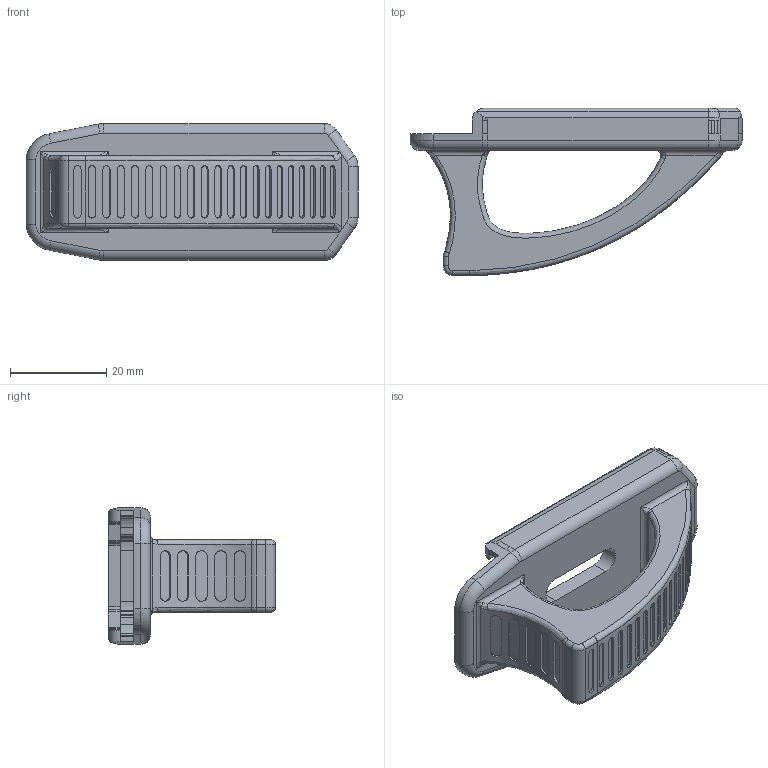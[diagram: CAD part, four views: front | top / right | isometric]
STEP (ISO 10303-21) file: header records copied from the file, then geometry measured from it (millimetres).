
FILE_DESCRIPTION (( 'STEP AP214' ), '1' );
FILE_NAME ('Ranger_Plate.STEP', '2022-09-24T15:52:26', ( '' ), ( '' ), 'SwSTEP 2.0', 'SolidWorks 2021', '' );
FILE_SCHEMA (( 'AUTOMOTIVE_DESIGN' ));
Length unit declared in the file: millimetre
Products named in the file (1): Ranger_Plate
Bounding box: 68.9 x 34.68 x 28.4 mm (x, y, z)
Volume: 15761.6 mm3; surface area: 8957.2 mm2
Topology: 1 solids, 1 shells, 302 faces, 759 edges, 478 vertices
Faces by surface type: bspline 118, plane 111, cylinder 59, torus 14
Entity records: 23687 total; most frequent: CARTESIAN_POINT 17571, ORIENTED_EDGE 1506, DIRECTION 827, EDGE_CURVE 753, VERTEX_POINT 478, B_SPLINE_CURVE_WITH_KNOTS 388, EDGE_LOOP 331, ADVANCED_FACE 302
